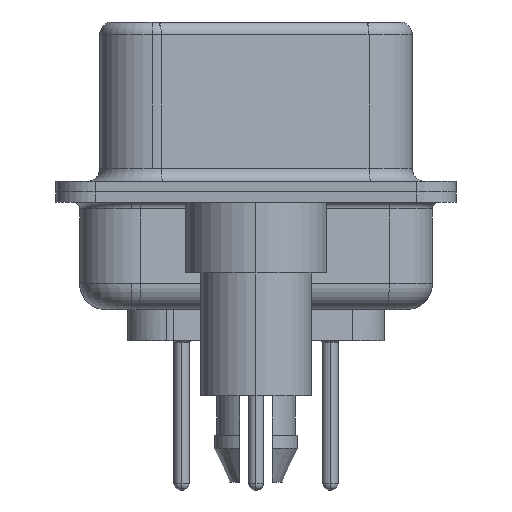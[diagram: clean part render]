
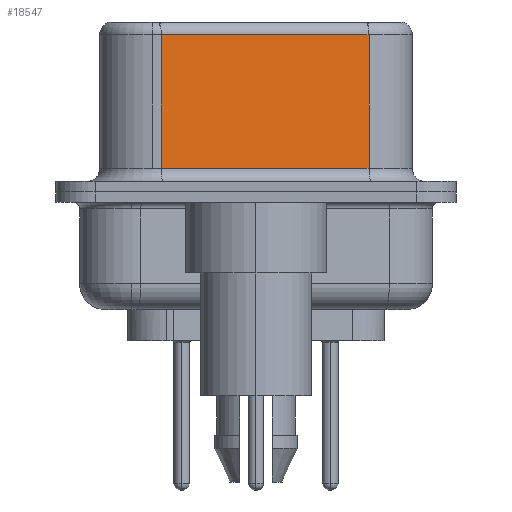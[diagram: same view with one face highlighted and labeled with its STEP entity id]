
A CAD part, left-side view. The second image highlights one B-rep face of the part: STEP entity #18547.
In plain terms, the highlighted planar face has unit normal (-0.985, -0.174, 0).
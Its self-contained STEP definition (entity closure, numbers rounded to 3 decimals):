
#311 = DIRECTION ( 'NONE',  ( -0.174, 0.985, 0. ) ) ;
#1483 = EDGE_LOOP ( 'NONE', ( #6653, #26440, #25356, #25557 ) ) ;
#2628 = CARTESIAN_POINT ( 'NONE',  ( 5.132, -4.322, 6.02 ) ) ;
#3157 = CARTESIAN_POINT ( 'NONE',  ( 3.73, 3.628, 0.9 ) ) ;
#3180 = FACE_OUTER_BOUND ( 'NONE', #1483, .T. ) ;
#4287 = EDGE_CURVE ( 'NONE', #20684, #30217, #4404, .T. ) ;
#4404 = LINE ( 'NONE', #11584, #11401 ) ;
#4878 = CARTESIAN_POINT ( 'NONE',  ( 5.132, -4.322, 0.9 ) ) ;
#4905 = CARTESIAN_POINT ( 'NONE',  ( 5.132, -4.322, 6.02 ) ) ;
#4910 = EDGE_CURVE ( 'NONE', #8622, #5696, #10414, .T. ) ;
#5696 = VERTEX_POINT ( 'NONE', #3157 ) ;
#6110 = AXIS2_PLACEMENT_3D ( 'NONE', #17097, #19549, #10209 ) ;
#6653 = ORIENTED_EDGE ( 'NONE', *, *, #4287, .F. ) ;
#8622 = VERTEX_POINT ( 'NONE', #24417 ) ;
#8720 = CARTESIAN_POINT ( 'NONE',  ( 5.132, -4.322, 0.9 ) ) ;
#9007 = VECTOR ( 'NONE', #17602, 1000. ) ;
#10209 = DIRECTION ( 'NONE',  ( -0.174, 0.985, 0. ) ) ;
#10414 = LINE ( 'NONE', #24634, #9007 ) ;
#11401 = VECTOR ( 'NONE', #18479, 1000. ) ;
#11403 = EDGE_CURVE ( 'NONE', #5696, #30217, #25833, .T. ) ;
#11584 = CARTESIAN_POINT ( 'NONE',  ( 5.132, -4.322, 6.52 ) ) ;
#15942 = VECTOR ( 'NONE', #311, 1000. ) ;
#17097 = CARTESIAN_POINT ( 'NONE',  ( 5.132, -4.322, 6.52 ) ) ;
#17602 = DIRECTION ( 'NONE',  ( 0., 0., -1. ) ) ;
#18479 = DIRECTION ( 'NONE',  ( 0., 0., -1. ) ) ;
#18547 = ADVANCED_FACE ( 'NONE', ( #3180 ), #22140, .F. ) ;
#19339 = EDGE_CURVE ( 'NONE', #20684, #8622, #28482, .T. ) ;
#19549 = DIRECTION ( 'NONE',  ( 0.985, 0.174, 0. ) ) ;
#20684 = VERTEX_POINT ( 'NONE', #4905 ) ;
#22140 = PLANE ( 'NONE',  #6110 ) ;
#22503 = VECTOR ( 'NONE', #23541, 1000. ) ;
#23541 = DIRECTION ( 'NONE',  ( 0.174, -0.985, 0. ) ) ;
#24417 = CARTESIAN_POINT ( 'NONE',  ( 3.73, 3.628, 6.02 ) ) ;
#24634 = CARTESIAN_POINT ( 'NONE',  ( 3.73, 3.628, 6.52 ) ) ;
#25356 = ORIENTED_EDGE ( 'NONE', *, *, #4910, .T. ) ;
#25557 = ORIENTED_EDGE ( 'NONE', *, *, #11403, .T. ) ;
#25833 = LINE ( 'NONE', #4878, #22503 ) ;
#26440 = ORIENTED_EDGE ( 'NONE', *, *, #19339, .T. ) ;
#28482 = LINE ( 'NONE', #2628, #15942 ) ;
#30217 = VERTEX_POINT ( 'NONE', #8720 ) ;
